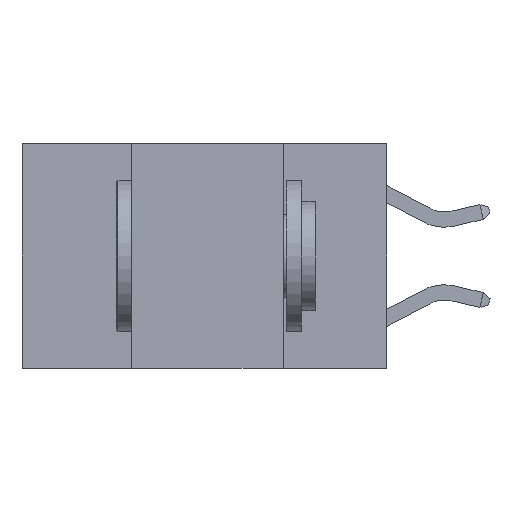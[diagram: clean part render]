
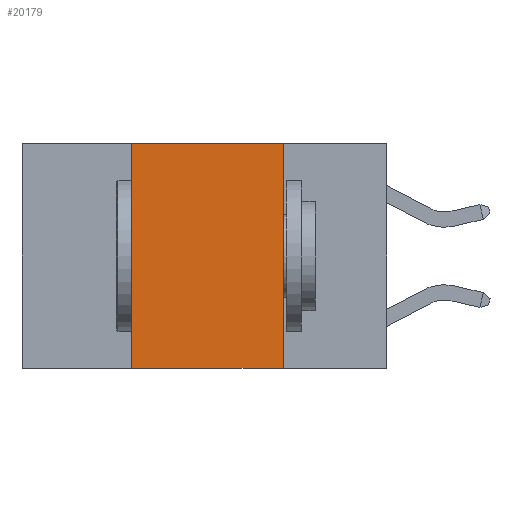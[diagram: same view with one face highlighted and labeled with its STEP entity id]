
A CAD part, left-side view. The second image highlights one B-rep face of the part: STEP entity #20179.
In plain terms, the highlighted planar face has unit normal (-1, 0, 0).
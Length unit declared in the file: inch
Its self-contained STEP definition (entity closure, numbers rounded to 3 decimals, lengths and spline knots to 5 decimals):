
#1372 = ORIENTED_EDGE ( 'NONE', *, *, #17607, .F. ) ;
#1432 = ORIENTED_EDGE ( 'NONE', *, *, #18705, .T. ) ;
#2662 = DIRECTION ( 'NONE',  ( 1., 0., 0. ) ) ;
#4922 = AXIS2_PLACEMENT_3D ( 'NONE', #10804, #2662, #8715 ) ;
#5103 = VERTEX_POINT ( 'NONE', #18861 ) ;
#6145 = VERTEX_POINT ( 'NONE', #18915 ) ;
#6435 = VERTEX_POINT ( 'NONE', #16808 ) ;
#7034 = CARTESIAN_POINT ( 'NONE',  ( 0., 0.6, -0.37 ) ) ;
#7563 = PLANE ( 'NONE',  #4922 ) ;
#8202 = DIRECTION ( 'NONE',  ( 0., -1., 0. ) ) ;
#8229 = VECTOR ( 'NONE', #8202, 39.37008 ) ;
#8715 = DIRECTION ( 'NONE',  ( 0., 0., -1. ) ) ;
#10457 = CARTESIAN_POINT ( 'NONE',  ( 0., 0.17, -0.37 ) ) ;
#10676 = CARTESIAN_POINT ( 'NONE',  ( 0., 0.42, 0. ) ) ;
#10804 = CARTESIAN_POINT ( 'NONE',  ( 0., 0.6, 0. ) ) ;
#11702 = DIRECTION ( 'NONE',  ( 0., -1., 0. ) ) ;
#12155 = CARTESIAN_POINT ( 'NONE',  ( 0., 0.17, 0. ) ) ;
#12235 = DIRECTION ( 'NONE',  ( 0., 0., 1. ) ) ;
#12893 = VECTOR ( 'NONE', #12235, 39.37008 ) ;
#13504 = FACE_OUTER_BOUND ( 'NONE', #20005, .T. ) ;
#13670 = LINE ( 'NONE', #14926, #14835 ) ;
#14100 = LINE ( 'NONE', #10676, #12893 ) ;
#14104 = LINE ( 'NONE', #12155, #19222 ) ;
#14835 = VECTOR ( 'NONE', #11702, 39.37008 ) ;
#14926 = CARTESIAN_POINT ( 'NONE',  ( 0., 0.6, 0. ) ) ;
#15692 = ORIENTED_EDGE ( 'NONE', *, *, #18853, .F. ) ;
#16088 = EDGE_CURVE ( 'NONE', #6145, #6435, #13670, .T. ) ;
#16114 = LINE ( 'NONE', #7034, #8229 ) ;
#16808 = CARTESIAN_POINT ( 'NONE',  ( 0., 0.17, 0. ) ) ;
#17583 = VERTEX_POINT ( 'NONE', #10457 ) ;
#17607 = EDGE_CURVE ( 'NONE', #5103, #6145, #14100, .T. ) ;
#18167 = DIRECTION ( 'NONE',  ( 0., 0., -1. ) ) ;
#18705 = EDGE_CURVE ( 'NONE', #5103, #17583, #16114, .T. ) ;
#18853 = EDGE_CURVE ( 'NONE', #6435, #17583, #14104, .T. ) ;
#18861 = CARTESIAN_POINT ( 'NONE',  ( 0., 0.42, -0.37 ) ) ;
#18915 = CARTESIAN_POINT ( 'NONE',  ( 0., 0.42, 0. ) ) ;
#19222 = VECTOR ( 'NONE', #18167, 39.37008 ) ;
#20005 = EDGE_LOOP ( 'NONE', ( #15692, #20162, #1372, #1432 ) ) ;
#20162 = ORIENTED_EDGE ( 'NONE', *, *, #16088, .F. ) ;
#20179 = ADVANCED_FACE ( 'NONE', ( #13504 ), #7563, .F. ) ;
